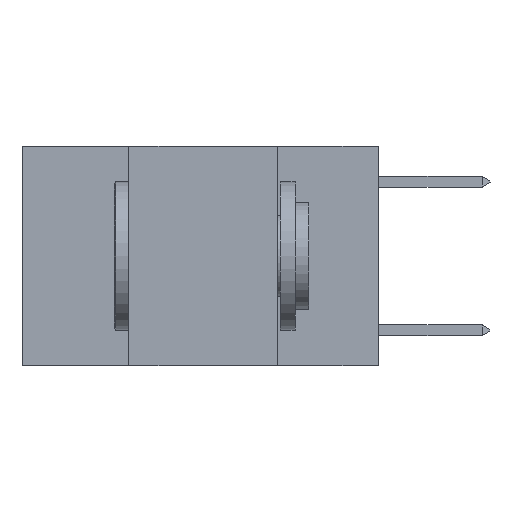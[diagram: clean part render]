
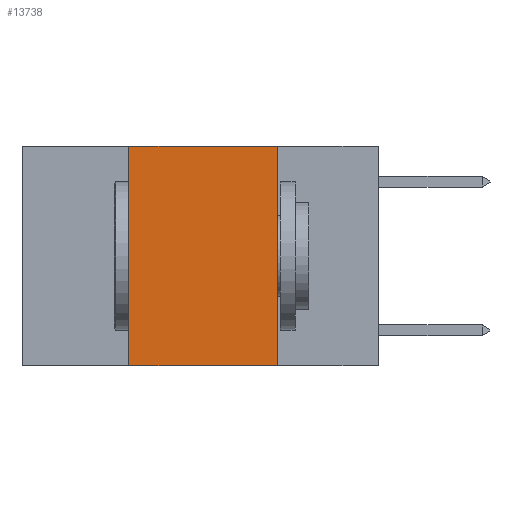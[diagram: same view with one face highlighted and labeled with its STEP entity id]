
A CAD part, left-side view. The second image highlights one B-rep face of the part: STEP entity #13738.
In plain terms, the highlighted planar face has unit normal (-1, 0, 0).
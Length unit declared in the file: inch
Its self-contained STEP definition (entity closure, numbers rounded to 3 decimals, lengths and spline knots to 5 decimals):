
#74 = EDGE_CURVE ( 'NONE', #8396, #358, #2133, .T. ) ;
#332 = ORIENTED_EDGE ( 'NONE', *, *, #10544, .F. ) ;
#358 = VERTEX_POINT ( 'NONE', #5651 ) ;
#411 = CARTESIAN_POINT ( 'NONE',  ( 0., 0.17, 0. ) ) ;
#1025 = VECTOR ( 'NONE', #13674, 39.37008 ) ;
#1766 = EDGE_LOOP ( 'NONE', ( #8795, #332, #9513, #12974 ) ) ;
#1889 = DIRECTION ( 'NONE',  ( 0., -1., 0. ) ) ;
#2133 = LINE ( 'NONE', #411, #1025 ) ;
#2158 = CARTESIAN_POINT ( 'NONE',  ( 0., 0.6, 0. ) ) ;
#3114 = CARTESIAN_POINT ( 'NONE',  ( 0., 0.6, -0.37 ) ) ;
#3309 = CARTESIAN_POINT ( 'NONE',  ( 0., 0.42, -0.37 ) ) ;
#3726 = CARTESIAN_POINT ( 'NONE',  ( 0., 0.42, 0. ) ) ;
#3797 = CARTESIAN_POINT ( 'NONE',  ( 0., 0.6, 0. ) ) ;
#5651 = CARTESIAN_POINT ( 'NONE',  ( 0., 0.17, -0.37 ) ) ;
#5822 = VECTOR ( 'NONE', #1889, 39.37008 ) ;
#6674 = DIRECTION ( 'NONE',  ( 0., 0., -1. ) ) ;
#6876 = FACE_OUTER_BOUND ( 'NONE', #1766, .T. ) ;
#7715 = LINE ( 'NONE', #15109, #7753 ) ;
#7753 = VECTOR ( 'NONE', #10691, 39.37008 ) ;
#8396 = VERTEX_POINT ( 'NONE', #13634 ) ;
#8795 = ORIENTED_EDGE ( 'NONE', *, *, #74, .F. ) ;
#9139 = DIRECTION ( 'NONE',  ( 0., -1., 0. ) ) ;
#9513 = ORIENTED_EDGE ( 'NONE', *, *, #14809, .F. ) ;
#9678 = AXIS2_PLACEMENT_3D ( 'NONE', #2158, #15854, #6674 ) ;
#9828 = LINE ( 'NONE', #3114, #19367 ) ;
#10544 = EDGE_CURVE ( 'NONE', #16442, #8396, #12700, .T. ) ;
#10691 = DIRECTION ( 'NONE',  ( 0., 0., 1. ) ) ;
#11027 = PLANE ( 'NONE',  #9678 ) ;
#11065 = EDGE_CURVE ( 'NONE', #17293, #358, #9828, .T. ) ;
#12700 = LINE ( 'NONE', #3797, #5822 ) ;
#12974 = ORIENTED_EDGE ( 'NONE', *, *, #11065, .T. ) ;
#13634 = CARTESIAN_POINT ( 'NONE',  ( 0., 0.17, 0. ) ) ;
#13674 = DIRECTION ( 'NONE',  ( 0., 0., -1. ) ) ;
#13738 = ADVANCED_FACE ( 'NONE', ( #6876 ), #11027, .F. ) ;
#14809 = EDGE_CURVE ( 'NONE', #17293, #16442, #7715, .T. ) ;
#15109 = CARTESIAN_POINT ( 'NONE',  ( 0., 0.42, 0. ) ) ;
#15854 = DIRECTION ( 'NONE',  ( 1., 0., 0. ) ) ;
#16442 = VERTEX_POINT ( 'NONE', #3726 ) ;
#17293 = VERTEX_POINT ( 'NONE', #3309 ) ;
#19367 = VECTOR ( 'NONE', #9139, 39.37008 ) ;
